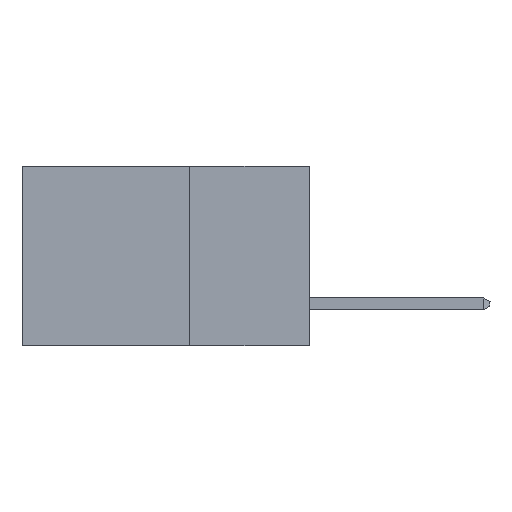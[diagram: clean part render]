
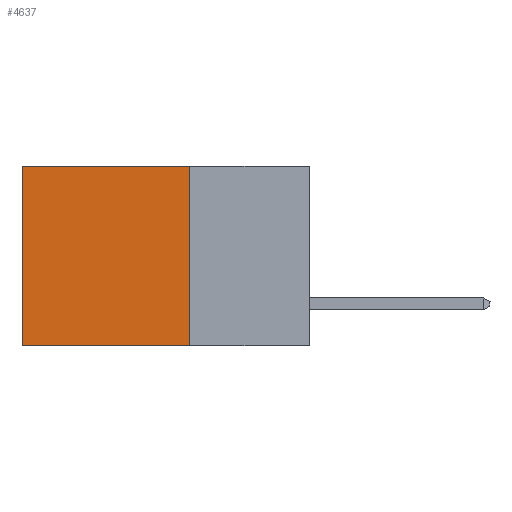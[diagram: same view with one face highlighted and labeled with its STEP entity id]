
A CAD part, left-side view. The second image highlights one B-rep face of the part: STEP entity #4637.
In plain terms, the highlighted planar face has unit normal (-1, 0, 0).
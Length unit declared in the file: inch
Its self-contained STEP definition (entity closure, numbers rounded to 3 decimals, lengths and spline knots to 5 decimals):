
#99 = LINE ( 'NONE', #2460, #3330 ) ;
#315 = CARTESIAN_POINT ( 'NONE',  ( 0.2875, 0.6, -0.375 ) ) ;
#353 = VERTEX_POINT ( 'NONE', #6863 ) ;
#557 = DIRECTION ( 'NONE',  ( 0., 0., -1. ) ) ;
#615 = CARTESIAN_POINT ( 'NONE',  ( 0.2875, 0.25, 0. ) ) ;
#685 = LINE ( 'NONE', #3757, #4345 ) ;
#764 = FACE_OUTER_BOUND ( 'NONE', #7508, .T. ) ;
#937 = CARTESIAN_POINT ( 'NONE',  ( 0.2875, 0.6, -0.375 ) ) ;
#942 = EDGE_CURVE ( 'NONE', #353, #6163, #99, .T. ) ;
#1069 = DIRECTION ( 'NONE',  ( 0., 1., 0. ) ) ;
#1622 = LINE ( 'NONE', #615, #8276 ) ;
#2460 = CARTESIAN_POINT ( 'NONE',  ( 0.2875, 0.25, -0.375 ) ) ;
#2503 = CARTESIAN_POINT ( 'NONE',  ( 0.2875, 0.25, -0.375 ) ) ;
#3036 = PLANE ( 'NONE',  #7824 ) ;
#3330 = VECTOR ( 'NONE', #557, 39.37008 ) ;
#3362 = DIRECTION ( 'NONE',  ( 0., 1., 0. ) ) ;
#3388 = ORIENTED_EDGE ( 'NONE', *, *, #5084, .T. ) ;
#3757 = CARTESIAN_POINT ( 'NONE',  ( 0.2875, 0.25, -0.375 ) ) ;
#3905 = EDGE_CURVE ( 'NONE', #6163, #4990, #685, .T. ) ;
#4227 = VERTEX_POINT ( 'NONE', #7790 ) ;
#4345 = VECTOR ( 'NONE', #1069, 39.37008 ) ;
#4424 = ORIENTED_EDGE ( 'NONE', *, *, #3905, .F. ) ;
#4474 = ORIENTED_EDGE ( 'NONE', *, *, #8108, .T. ) ;
#4637 = ADVANCED_FACE ( 'NONE', ( #764 ), #3036, .F. ) ;
#4990 = VERTEX_POINT ( 'NONE', #315 ) ;
#5084 = EDGE_CURVE ( 'NONE', #4227, #4990, #6020, .T. ) ;
#5577 = DIRECTION ( 'NONE',  ( 0., 0., -1. ) ) ;
#5619 = VECTOR ( 'NONE', #5577, 39.37008 ) ;
#5636 = DIRECTION ( 'NONE',  ( 1., 0., 0. ) ) ;
#6020 = LINE ( 'NONE', #937, #5619 ) ;
#6163 = VERTEX_POINT ( 'NONE', #2503 ) ;
#6171 = ORIENTED_EDGE ( 'NONE', *, *, #942, .F. ) ;
#6282 = DIRECTION ( 'NONE',  ( 0., 0., -1. ) ) ;
#6327 = CARTESIAN_POINT ( 'NONE',  ( 0.2875, 0.25, -0.375 ) ) ;
#6863 = CARTESIAN_POINT ( 'NONE',  ( 0.2875, 0.25, 0. ) ) ;
#7508 = EDGE_LOOP ( 'NONE', ( #3388, #4424, #6171, #4474 ) ) ;
#7790 = CARTESIAN_POINT ( 'NONE',  ( 0.2875, 0.6, 0. ) ) ;
#7824 = AXIS2_PLACEMENT_3D ( 'NONE', #6327, #5636, #6282 ) ;
#8108 = EDGE_CURVE ( 'NONE', #353, #4227, #1622, .T. ) ;
#8276 = VECTOR ( 'NONE', #3362, 39.37008 ) ;
